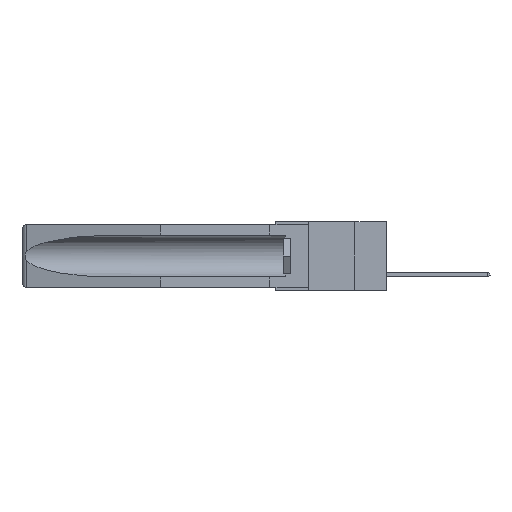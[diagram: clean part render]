
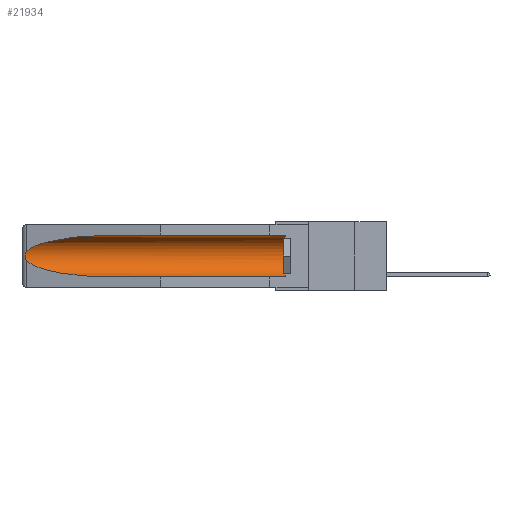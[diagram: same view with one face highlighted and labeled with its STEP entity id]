
A CAD part, left-side view. The second image highlights one B-rep face of the part: STEP entity #21934.
In plain terms, the highlighted cylindrical face has radius 2.857 mm (diameter 5.715 mm), a partial arc.
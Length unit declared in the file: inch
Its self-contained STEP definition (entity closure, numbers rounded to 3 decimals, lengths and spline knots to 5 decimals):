
#797 = VERTEX_POINT ( 'NONE', #11548 ) ;
#932 = CARTESIAN_POINT ( 'NONE',  ( 0.2675, 1.53308, -0.16763 ) ) ;
#978 = EDGE_CURVE ( 'NONE', #11747, #2942, #14604, .T. ) ;
#1045 = CARTESIAN_POINT ( 'NONE',  ( 0.26597, 1.5296, -0.19026 ) ) ;
#1470 = CARTESIAN_POINT ( 'NONE',  ( 0.155, 1.07973, -0.059 ) ) ;
#1583 = CARTESIAN_POINT ( 'NONE',  ( 0.155, 1.07973, -0.284 ) ) ;
#1826 = VECTOR ( 'NONE', #23622, 39.37008 ) ;
#1927 = CARTESIAN_POINT ( 'NONE',  ( 0.155, 1.07973, -0.284 ) ) ;
#2189 = EDGE_CURVE ( 'NONE', #9052, #10599, #8844, .T. ) ;
#2246 = CARTESIAN_POINT ( 'NONE',  ( 0.21114, 1.30732, -0.284 ) ) ;
#2315 = CARTESIAN_POINT ( 'NONE',  ( 0.21114, 1.30732, -0.059 ) ) ;
#2942 = VERTEX_POINT ( 'NONE', #12631 ) ;
#3404 = CARTESIAN_POINT ( 'NONE',  ( 0.2675, 1.53308, -0.17534 ) ) ;
#3500 = CARTESIAN_POINT ( 'NONE',  ( 0.26654, 1.53092, -0.15636 ) ) ;
#4717 = DIRECTION ( 'NONE',  ( 0., 1., 0. ) ) ;
#5967 = CARTESIAN_POINT ( 'NONE',  ( 0.26537, 1.52718, -0.19328 ) ) ;
#6537 = ORIENTED_EDGE ( 'NONE', *, *, #17445, .T. ) ;
#6849 = CARTESIAN_POINT ( 'NONE',  ( 0.25451, 1.48313, -0.24835 ) ) ;
#7195 = EDGE_CURVE ( 'NONE', #797, #11747, #13757, .T. ) ;
#7196 = DIRECTION ( 'NONE',  ( 0., 0., 1. ) ) ;
#8844 =( BOUNDED_CURVE ( )  B_SPLINE_CURVE ( 3, ( #17005, #6849, #2246, #1927 ),
 .UNSPECIFIED., .F., .F. ) 
 B_SPLINE_CURVE_WITH_KNOTS ( ( 4, 4 ),
 ( 0.1948, 1.5708 ),
 .UNSPECIFIED. ) 
 CURVE ( )  GEOMETRIC_REPRESENTATION_ITEM ( )  RATIONAL_B_SPLINE_CURVE ( ( 1., 0.848, 0.848, 1. ) ) 
 REPRESENTATION_ITEM ( '' )  );
#9021 = ORIENTED_EDGE ( 'NONE', *, *, #978, .T. ) ;
#9052 = VERTEX_POINT ( 'NONE', #17020 ) ;
#9339 = EDGE_LOOP ( 'NONE', ( #9021, #6537, #10832, #31074, #16195, #26279 ) ) ;
#9583 = CARTESIAN_POINT ( 'NONE',  ( 0.155, 1.07973, -0.059 ) ) ;
#10599 = VERTEX_POINT ( 'NONE', #1583 ) ;
#10832 = ORIENTED_EDGE ( 'NONE', *, *, #2189, .T. ) ;
#10906 = CARTESIAN_POINT ( 'NONE',  ( 0.26537, 1.52718, -0.14972 ) ) ;
#11077 = DIRECTION ( 'NONE',  ( 0., -1., 0. ) ) ;
#11132 = CARTESIAN_POINT ( 'NONE',  ( 0.155, -0.30754, -0.059 ) ) ;
#11548 = CARTESIAN_POINT ( 'NONE',  ( 0.155, 0.126, -0.059 ) ) ;
#11747 = VERTEX_POINT ( 'NONE', #1470 ) ;
#12631 = CARTESIAN_POINT ( 'NONE',  ( 0.26537, 1.52718, -0.14972 ) ) ;
#13489 = CARTESIAN_POINT ( 'NONE',  ( 0.2673, 1.5327, -0.16383 ) ) ;
#13596 = CARTESIAN_POINT ( 'NONE',  ( 0.26655, 1.53094, -0.18657 ) ) ;
#13757 = LINE ( 'NONE', #11132, #1826 ) ;
#13882 = DIRECTION ( 'NONE',  ( 0., 0., 1. ) ) ;
#14514 = EDGE_CURVE ( 'NONE', #16983, #10599, #28713, .T. ) ;
#14604 =( BOUNDED_CURVE ( )  B_SPLINE_CURVE ( 3, ( #9583, #2315, #26997, #19544 ),
 .UNSPECIFIED., .F., .F. ) 
 B_SPLINE_CURVE_WITH_KNOTS ( ( 4, 4 ),
 ( 4.71239, 6.08839 ),
 .UNSPECIFIED. ) 
 CURVE ( )  GEOMETRIC_REPRESENTATION_ITEM ( )  RATIONAL_B_SPLINE_CURVE ( ( 1., 0.848, 0.848, 1. ) ) 
 REPRESENTATION_ITEM ( '' )  );
#15575 = CARTESIAN_POINT ( 'NONE',  ( 0.155, -0.30754, -0.284 ) ) ;
#15786 = DIRECTION ( 'NONE',  ( 0., 1., 0. ) ) ;
#16195 = ORIENTED_EDGE ( 'NONE', *, *, #20106, .T. ) ;
#16283 = CARTESIAN_POINT ( 'NONE',  ( 0.155, 0.126, -0.1715 ) ) ;
#16983 = VERTEX_POINT ( 'NONE', #27611 ) ;
#17005 = CARTESIAN_POINT ( 'NONE',  ( 0.26537, 1.52718, -0.19328 ) ) ;
#17020 = CARTESIAN_POINT ( 'NONE',  ( 0.26537, 1.52718, -0.19328 ) ) ;
#17445 = EDGE_CURVE ( 'NONE', #2942, #9052, #22495, .T. ) ;
#18151 = CARTESIAN_POINT ( 'NONE',  ( 0.2673, 1.53269, -0.17917 ) ) ;
#19544 = CARTESIAN_POINT ( 'NONE',  ( 0.26537, 1.52718, -0.14972 ) ) ;
#20106 = EDGE_CURVE ( 'NONE', #16983, #797, #30387, .T. ) ;
#20820 = CARTESIAN_POINT ( 'NONE',  ( 0.26597, 1.52961, -0.15275 ) ) ;
#21934 = ADVANCED_FACE ( 'NONE', ( #24134 ), #24930, .F. ) ;
#22495 = B_SPLINE_CURVE_WITH_KNOTS ( 'NONE', 3,
 ( #10906, #20820, #3500, #13489, #932, #3404, #18151, #13596, #1045, #5967 ),
 .UNSPECIFIED., .F., .F.,
 ( 4, 2, 2, 2, 4 ),
 ( 0., 0.00029, 0.00058, 0.00087, 0.00117 ),
 .UNSPECIFIED. ) ;
#23622 = DIRECTION ( 'NONE',  ( 0., 1., 0. ) ) ;
#24134 = FACE_OUTER_BOUND ( 'NONE', #9339, .T. ) ;
#24930 = CYLINDRICAL_SURFACE ( 'NONE', #29206, 0.1125 ) ;
#25202 = AXIS2_PLACEMENT_3D ( 'NONE', #16283, #11077, #13882 ) ;
#26279 = ORIENTED_EDGE ( 'NONE', *, *, #7195, .T. ) ;
#26362 = VECTOR ( 'NONE', #15786, 39.37008 ) ;
#26997 = CARTESIAN_POINT ( 'NONE',  ( 0.25451, 1.48313, -0.09465 ) ) ;
#27282 = CARTESIAN_POINT ( 'NONE',  ( 0.155, -0.30754, -0.1715 ) ) ;
#27611 = CARTESIAN_POINT ( 'NONE',  ( 0.155, 0.126, -0.284 ) ) ;
#28713 = LINE ( 'NONE', #15575, #26362 ) ;
#29206 = AXIS2_PLACEMENT_3D ( 'NONE', #27282, #4717, #7196 ) ;
#30387 = CIRCLE ( 'NONE', #25202, 0.1125 ) ;
#31074 = ORIENTED_EDGE ( 'NONE', *, *, #14514, .F. ) ;
